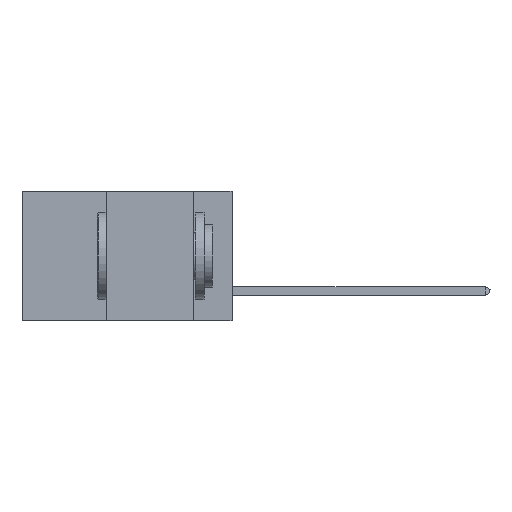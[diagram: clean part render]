
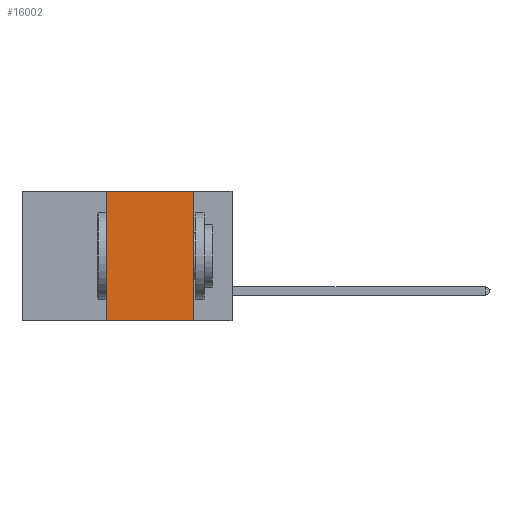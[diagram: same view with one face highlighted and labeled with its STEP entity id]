
A CAD part, left-side view. The second image highlights one B-rep face of the part: STEP entity #16002.
In plain terms, the highlighted planar face has unit normal (-1, 0, 0).
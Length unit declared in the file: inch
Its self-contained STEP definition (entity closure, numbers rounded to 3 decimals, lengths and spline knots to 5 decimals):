
#485 = VERTEX_POINT ( 'NONE', #42823 ) ;
#5025 = CARTESIAN_POINT ( 'NONE',  ( 0., 0.36, 0. ) ) ;
#5626 = CARTESIAN_POINT ( 'NONE',  ( 0., 0.36, 0. ) ) ;
#8470 = DIRECTION ( 'NONE',  ( 0., -1., 0. ) ) ;
#9037 = ORIENTED_EDGE ( 'NONE', *, *, #24494, .F. ) ;
#13728 = LINE ( 'NONE', #23493, #35178 ) ;
#15343 = VERTEX_POINT ( 'NONE', #40426 ) ;
#16002 = ADVANCED_FACE ( 'NONE', ( #27807 ), #43180, .F. ) ;
#17044 = VECTOR ( 'NONE', #24386, 39.37008 ) ;
#17111 = DIRECTION ( 'NONE',  ( 0., 0., -1. ) ) ;
#19316 = LINE ( 'NONE', #5626, #17044 ) ;
#20432 = LINE ( 'NONE', #39984, #27438 ) ;
#22424 = VERTEX_POINT ( 'NONE', #5025 ) ;
#23260 = EDGE_LOOP ( 'NONE', ( #34356, #9037, #43171, #36718 ) ) ;
#23493 = CARTESIAN_POINT ( 'NONE',  ( 0., 0.6, -0.37 ) ) ;
#24386 = DIRECTION ( 'NONE',  ( 0., 0., 1. ) ) ;
#24494 = EDGE_CURVE ( 'NONE', #22424, #485, #30369, .T. ) ;
#26147 = EDGE_CURVE ( 'NONE', #41655, #22424, #19316, .T. ) ;
#27438 = VECTOR ( 'NONE', #32357, 39.37008 ) ;
#27807 = FACE_OUTER_BOUND ( 'NONE', #23260, .T. ) ;
#29060 = DIRECTION ( 'NONE',  ( 0., -1., 0. ) ) ;
#30239 = EDGE_CURVE ( 'NONE', #41655, #15343, #13728, .T. ) ;
#30369 = LINE ( 'NONE', #40540, #42572 ) ;
#31959 = DIRECTION ( 'NONE',  ( 1., 0., 0. ) ) ;
#32357 = DIRECTION ( 'NONE',  ( 0., 0., -1. ) ) ;
#34356 = ORIENTED_EDGE ( 'NONE', *, *, #48214, .F. ) ;
#35178 = VECTOR ( 'NONE', #8470, 39.37008 ) ;
#36718 = ORIENTED_EDGE ( 'NONE', *, *, #30239, .T. ) ;
#39984 = CARTESIAN_POINT ( 'NONE',  ( 0., 0.11, 0. ) ) ;
#40426 = CARTESIAN_POINT ( 'NONE',  ( 0., 0.11, -0.37 ) ) ;
#40540 = CARTESIAN_POINT ( 'NONE',  ( 0., 0.6, 0. ) ) ;
#41094 = CARTESIAN_POINT ( 'NONE',  ( 0., 0.36, -0.37 ) ) ;
#41655 = VERTEX_POINT ( 'NONE', #41094 ) ;
#42572 = VECTOR ( 'NONE', #29060, 39.37008 ) ;
#42823 = CARTESIAN_POINT ( 'NONE',  ( 0., 0.11, 0. ) ) ;
#42990 = CARTESIAN_POINT ( 'NONE',  ( 0., 0.6, 0. ) ) ;
#43171 = ORIENTED_EDGE ( 'NONE', *, *, #26147, .F. ) ;
#43180 = PLANE ( 'NONE',  #43246 ) ;
#43246 = AXIS2_PLACEMENT_3D ( 'NONE', #42990, #31959, #17111 ) ;
#48214 = EDGE_CURVE ( 'NONE', #485, #15343, #20432, .T. ) ;
